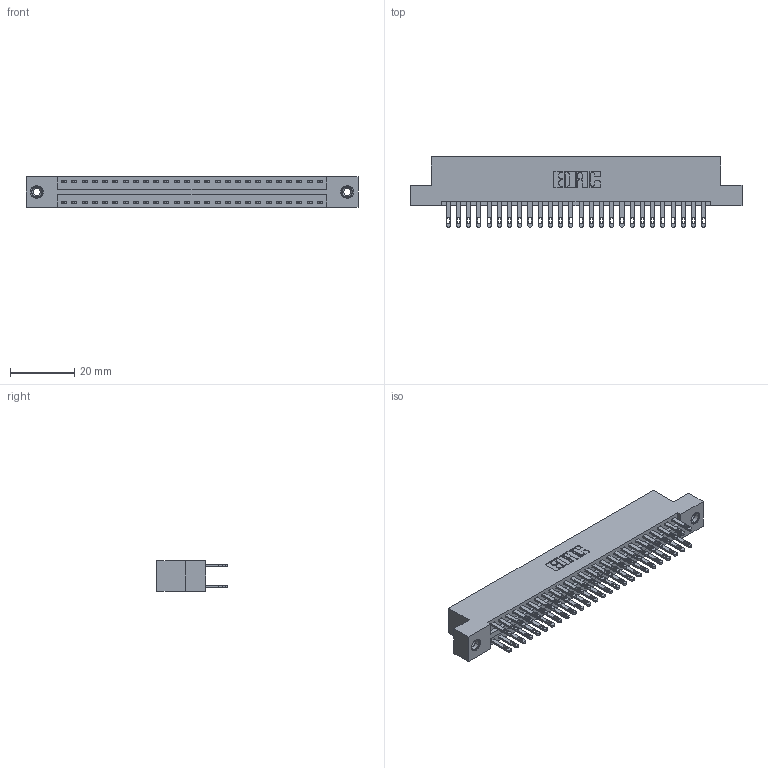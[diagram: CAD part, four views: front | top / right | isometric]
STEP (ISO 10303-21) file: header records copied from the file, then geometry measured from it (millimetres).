
FILE_DESCRIPTION (( 'STEP AP203' ), '1' );
FILE_NAME ('896-052-500-208.STEP', '2021-07-27T23:45:01', ( '' ), ( '' ), 'SwSTEP 2.0', 'SolidWorks 2020', '' );
FILE_SCHEMA (( 'CONFIG_CONTROL_DESIGN' ));
Length unit declared in the file: inch
Products named in the file (4): 345-250-001_345-250-003-102; 846 Part_Flush Mounting Lugs - 0.156 Dia-TI; 896-052-500-208; 345-292-001_345-293-100
Assembly tree (55 placements, depth 2):
  896-052-500-208
    846 Part_Flush Mounting Lugs - 0.156 Dia-TI
    345-292-001_345-293-100  x52
    345-250-001_345-250-003-102  x2
Bounding box: 103.12 x 21.84 x 9.4 mm (x, y, z)
Volume: 10084 mm3; surface area: 14173.9 mm2
Topology: 55 solids, 55 shells, 2678 faces, 8109 edges, 5398 vertices
Faces by surface type: plane 1616, cylinder 1046, cone 12, torus 4
Entity records: 20238 total; most frequent: CARTESIAN_POINT 3339, ORIENTED_EDGE 3266, DIRECTION 3023, EDGE_CURVE 1633, LINE 1373, VECTOR 1373, VERTEX_POINT 1084, AXIS2_PLACEMENT_3D 825
